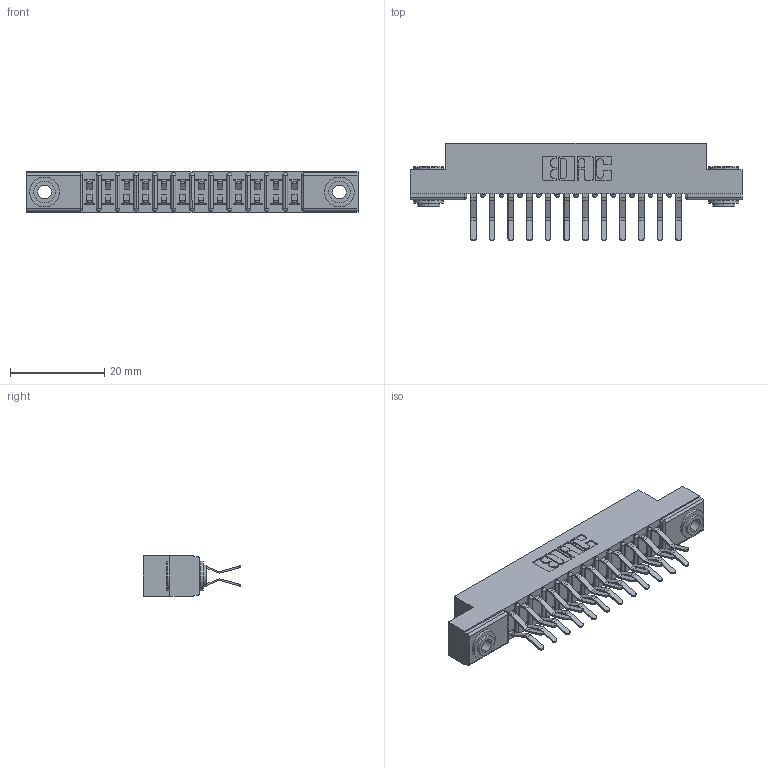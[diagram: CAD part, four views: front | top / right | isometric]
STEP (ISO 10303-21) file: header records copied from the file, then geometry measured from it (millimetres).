
FILE_DESCRIPTION (( 'STEP AP203' ), '1' );
FILE_NAME ('307-024-560-203.STEP', '2019-09-05T22:34:16', ( '' ), ( '' ), 'SwSTEP 2.0', 'SolidWorks 2016', '' );
FILE_SCHEMA (( 'CONFIG_CONTROL_DESIGN' ));
Length unit declared in the file: inch
Products named in the file (4): 307-024-560-203; 307-290-001_560; 345-250-002_345-250-002-102; 307 Part_.156 Dia Mounting Holes
Assembly tree (27 placements, depth 2):
  307-024-560-203
    307 Part_.156 Dia Mounting Holes
    307-290-001_560  x24
    345-250-002_345-250-002-102  x2
Bounding box: 70.56 x 20.73 x 8.71 mm (x, y, z)
Volume: 4647.8 mm3; surface area: 8116.6 mm2
Topology: 27 solids, 27 shells, 1383 faces, 3843 edges, 2490 vertices
Faces by surface type: plane 886, cylinder 463, sphere 26, cone 8
Entity records: 15539 total; most frequent: CARTESIAN_POINT 2533, DIRECTION 2509, ORIENTED_EDGE 2498, EDGE_CURVE 1249, VECTOR 937, LINE 937, VERTEX_POINT 810, AXIS2_PLACEMENT_3D 786
